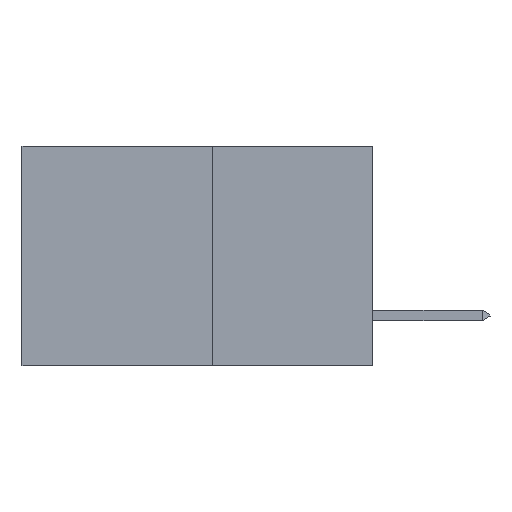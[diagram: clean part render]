
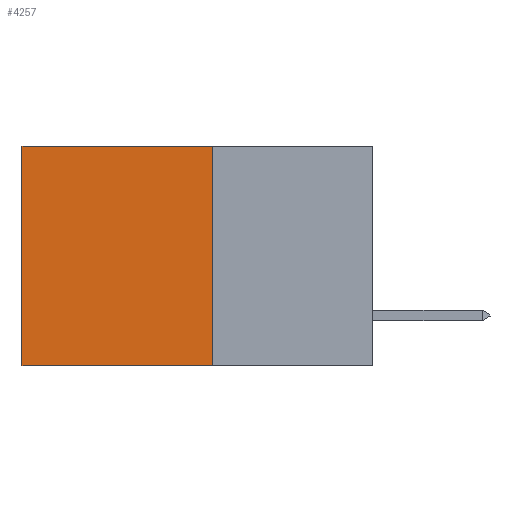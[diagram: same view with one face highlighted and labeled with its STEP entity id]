
A CAD part, left-side view. The second image highlights one B-rep face of the part: STEP entity #4257.
In plain terms, the highlighted planar face has unit normal (-1, 0, 0).
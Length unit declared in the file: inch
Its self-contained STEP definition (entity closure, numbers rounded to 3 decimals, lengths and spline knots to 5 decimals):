
#501 = EDGE_LOOP ( 'NONE', ( #12112, #20826, #17966, #10925 ) ) ;
#2349 = EDGE_CURVE ( 'NONE', #16612, #21424, #18737, .T. ) ;
#2528 = LINE ( 'NONE', #12125, #12527 ) ;
#3850 = DIRECTION ( 'NONE',  ( 0., 0., -1. ) ) ;
#4257 = ADVANCED_FACE ( 'NONE', ( #17152 ), #20240, .F. ) ;
#5229 = VECTOR ( 'NONE', #5270, 39.37008 ) ;
#5270 = DIRECTION ( 'NONE',  ( 0., 1., 0. ) ) ;
#5696 = VERTEX_POINT ( 'NONE', #23178 ) ;
#7410 = CARTESIAN_POINT ( 'NONE',  ( 0.277, 0.27, -0.37 ) ) ;
#7851 = DIRECTION ( 'NONE',  ( 0., 0., -1. ) ) ;
#7887 = DIRECTION ( 'NONE',  ( 1., 0., 0. ) ) ;
#9673 = CARTESIAN_POINT ( 'NONE',  ( 0.277, 0.59, -0.37 ) ) ;
#10925 = ORIENTED_EDGE ( 'NONE', *, *, #20764, .T. ) ;
#11177 = CARTESIAN_POINT ( 'NONE',  ( 0.277, 0.27, -0.37 ) ) ;
#11676 = VERTEX_POINT ( 'NONE', #11177 ) ;
#12112 = ORIENTED_EDGE ( 'NONE', *, *, #2349, .T. ) ;
#12125 = CARTESIAN_POINT ( 'NONE',  ( 0.277, 0.27, -0.37 ) ) ;
#12527 = VECTOR ( 'NONE', #23372, 39.37008 ) ;
#14582 = EDGE_CURVE ( 'NONE', #11676, #21424, #21035, .T. ) ;
#15194 = LINE ( 'NONE', #16415, #5229 ) ;
#16415 = CARTESIAN_POINT ( 'NONE',  ( 0.277, 0.27, 0. ) ) ;
#16612 = VERTEX_POINT ( 'NONE', #17021 ) ;
#16616 = VECTOR ( 'NONE', #18621, 39.37008 ) ;
#16706 = CARTESIAN_POINT ( 'NONE',  ( 0.277, 0.59, -0.37 ) ) ;
#17021 = CARTESIAN_POINT ( 'NONE',  ( 0.277, 0.59, 0. ) ) ;
#17152 = FACE_OUTER_BOUND ( 'NONE', #501, .T. ) ;
#17966 = ORIENTED_EDGE ( 'NONE', *, *, #23795, .F. ) ;
#18621 = DIRECTION ( 'NONE',  ( 0., 1., 0. ) ) ;
#18737 = LINE ( 'NONE', #9673, #23188 ) ;
#19510 = AXIS2_PLACEMENT_3D ( 'NONE', #20346, #7887, #7851 ) ;
#20240 = PLANE ( 'NONE',  #19510 ) ;
#20346 = CARTESIAN_POINT ( 'NONE',  ( 0.277, 0.27, -0.37 ) ) ;
#20764 = EDGE_CURVE ( 'NONE', #5696, #16612, #15194, .T. ) ;
#20826 = ORIENTED_EDGE ( 'NONE', *, *, #14582, .F. ) ;
#21035 = LINE ( 'NONE', #7410, #16616 ) ;
#21424 = VERTEX_POINT ( 'NONE', #16706 ) ;
#23178 = CARTESIAN_POINT ( 'NONE',  ( 0.277, 0.27, 0. ) ) ;
#23188 = VECTOR ( 'NONE', #3850, 39.37008 ) ;
#23372 = DIRECTION ( 'NONE',  ( 0., 0., -1. ) ) ;
#23795 = EDGE_CURVE ( 'NONE', #5696, #11676, #2528, .T. ) ;
